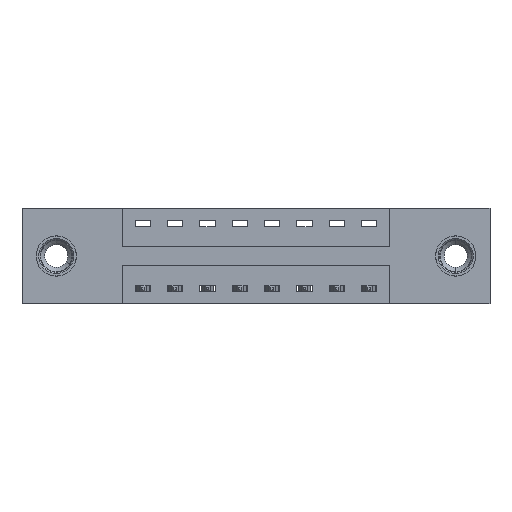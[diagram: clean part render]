
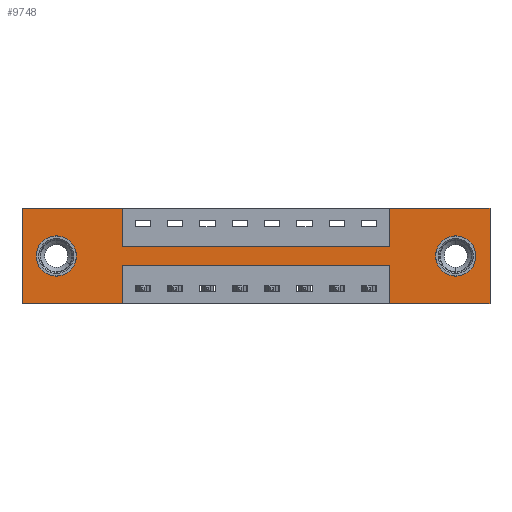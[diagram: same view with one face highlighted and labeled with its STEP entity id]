
A CAD part, front view. The second image highlights one B-rep face of the part: STEP entity #9748.
In plain terms, the highlighted planar face has unit normal (0, -1, 0).
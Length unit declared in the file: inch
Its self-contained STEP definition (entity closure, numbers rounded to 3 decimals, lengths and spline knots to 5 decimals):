
#38 = VERTEX_POINT ( 'NONE', #6421 ) ;
#64 = EDGE_LOOP ( 'NONE', ( #5988, #2363 ) ) ;
#204 = LINE ( 'NONE', #2705, #6734 ) ;
#238 = CARTESIAN_POINT ( 'NONE',  ( 0.3875, 0., -0.22 ) ) ;
#271 = LINE ( 'NONE', #597, #4645 ) ;
#382 = ORIENTED_EDGE ( 'NONE', *, *, #5666, .F. ) ;
#433 = EDGE_CURVE ( 'NONE', #2110, #8486, #7296, .T. ) ;
#437 = CARTESIAN_POINT ( 'NONE',  ( 0., 0., 0. ) ) ;
#597 = CARTESIAN_POINT ( 'NONE',  ( 0.3875, 0., -0.37 ) ) ;
#605 = CARTESIAN_POINT ( 'NONE',  ( 1.6775, 0., -0.185 ) ) ;
#645 = LINE ( 'NONE', #3397, #930 ) ;
#767 = EDGE_CURVE ( 'NONE', #38, #3267, #10589, .T. ) ;
#905 = VERTEX_POINT ( 'NONE', #4752 ) ;
#921 = ORIENTED_EDGE ( 'NONE', *, *, #1501, .F. ) ;
#930 = VECTOR ( 'NONE', #9151, 39.37008 ) ;
#946 = ORIENTED_EDGE ( 'NONE', *, *, #3650, .F. ) ;
#1101 = VECTOR ( 'NONE', #7994, 39.37008 ) ;
#1183 = VERTEX_POINT ( 'NONE', #7125 ) ;
#1222 = AXIS2_PLACEMENT_3D ( 'NONE', #1968, #10195, #5413 ) ;
#1232 = VECTOR ( 'NONE', #1485, 39.37008 ) ;
#1287 = AXIS2_PLACEMENT_3D ( 'NONE', #2606, #8405, #3456 ) ;
#1337 = ORIENTED_EDGE ( 'NONE', *, *, #9302, .F. ) ;
#1341 = FACE_BOUND ( 'NONE', #9958, .T. ) ;
#1353 = CARTESIAN_POINT ( 'NONE',  ( 1.81, 0., 0. ) ) ;
#1474 = ORIENTED_EDGE ( 'NONE', *, *, #5141, .F. ) ;
#1485 = DIRECTION ( 'NONE',  ( 1., 0., 0. ) ) ;
#1493 = DIRECTION ( 'NONE',  ( 0., 0., -1. ) ) ;
#1501 = EDGE_CURVE ( 'NONE', #9305, #10160, #5220, .T. ) ;
#1562 = CARTESIAN_POINT ( 'NONE',  ( 0.3875, 0., -0.22 ) ) ;
#1576 = VERTEX_POINT ( 'NONE', #10433 ) ;
#1651 = VECTOR ( 'NONE', #6190, 39.37008 ) ;
#1661 = AXIS2_PLACEMENT_3D ( 'NONE', #4784, #10378, #5609 ) ;
#1804 = DIRECTION ( 'NONE',  ( 0., 0., 1. ) ) ;
#1968 = CARTESIAN_POINT ( 'NONE',  ( 0., 0., -0.37 ) ) ;
#2008 = ORIENTED_EDGE ( 'NONE', *, *, #767, .F. ) ;
#2110 = VERTEX_POINT ( 'NONE', #6251 ) ;
#2145 = CARTESIAN_POINT ( 'NONE',  ( 1.4225, 0., -0.37 ) ) ;
#2183 = ORIENTED_EDGE ( 'NONE', *, *, #8426, .F. ) ;
#2271 = DIRECTION ( 'NONE',  ( 1., 0., 0. ) ) ;
#2363 = ORIENTED_EDGE ( 'NONE', *, *, #6330, .T. ) ;
#2386 = CARTESIAN_POINT ( 'NONE',  ( 1.4225, 0., -0.22 ) ) ;
#2452 = VERTEX_POINT ( 'NONE', #8284 ) ;
#2469 = DIRECTION ( 'NONE',  ( 0., 1., 0. ) ) ;
#2606 = CARTESIAN_POINT ( 'NONE',  ( 0.1325, 0., -0.185 ) ) ;
#2697 = VERTEX_POINT ( 'NONE', #9486 ) ;
#2705 = CARTESIAN_POINT ( 'NONE',  ( 0., 0., 0. ) ) ;
#2707 = CARTESIAN_POINT ( 'NONE',  ( 0.3875, 0., 0. ) ) ;
#2817 = CIRCLE ( 'NONE', #1661, 0.078 ) ;
#2905 = ORIENTED_EDGE ( 'NONE', *, *, #5493, .F. ) ;
#3236 = EDGE_CURVE ( 'NONE', #1576, #4786, #9096, .T. ) ;
#3246 = AXIS2_PLACEMENT_3D ( 'NONE', #7494, #2469, #8277 ) ;
#3267 = VERTEX_POINT ( 'NONE', #7894 ) ;
#3397 = CARTESIAN_POINT ( 'NONE',  ( 1.4225, 0., 0. ) ) ;
#3455 = VECTOR ( 'NONE', #5183, 39.37008 ) ;
#3456 = DIRECTION ( 'NONE',  ( 0., 0., 1. ) ) ;
#3497 = EDGE_CURVE ( 'NONE', #2697, #905, #6804, .T. ) ;
#3650 = EDGE_CURVE ( 'NONE', #10160, #2110, #5708, .T. ) ;
#3912 = CARTESIAN_POINT ( 'NONE',  ( 0., 0., -0.37 ) ) ;
#4524 = VECTOR ( 'NONE', #4642, 39.37008 ) ;
#4527 = CARTESIAN_POINT ( 'NONE',  ( 0., 0., -0.37 ) ) ;
#4559 = VECTOR ( 'NONE', #6404, 39.37008 ) ;
#4587 = PLANE ( 'NONE',  #1222 ) ;
#4642 = DIRECTION ( 'NONE',  ( -1., 0., 0. ) ) ;
#4645 = VECTOR ( 'NONE', #10512, 39.37008 ) ;
#4752 = CARTESIAN_POINT ( 'NONE',  ( 1.6775, 0., -0.263 ) ) ;
#4784 = CARTESIAN_POINT ( 'NONE',  ( 0.1325, 0., -0.185 ) ) ;
#4786 = VERTEX_POINT ( 'NONE', #4527 ) ;
#5141 = EDGE_CURVE ( 'NONE', #10484, #1576, #271, .T. ) ;
#5183 = DIRECTION ( 'NONE',  ( 0., 0., -1. ) ) ;
#5215 = EDGE_CURVE ( 'NONE', #1183, #6131, #8218, .T. ) ;
#5220 = LINE ( 'NONE', #6111, #9248 ) ;
#5273 = CARTESIAN_POINT ( 'NONE',  ( 0.3875, 0., -0.15 ) ) ;
#5409 = EDGE_CURVE ( 'NONE', #6879, #10484, #6156, .T. ) ;
#5413 = DIRECTION ( 'NONE',  ( 0., 0., -1. ) ) ;
#5493 = EDGE_CURVE ( 'NONE', #2452, #6879, #7342, .T. ) ;
#5609 = DIRECTION ( 'NONE',  ( 0., 0., 1. ) ) ;
#5666 = EDGE_CURVE ( 'NONE', #7062, #38, #10026, .T. ) ;
#5708 = LINE ( 'NONE', #9967, #3455 ) ;
#5742 = ORIENTED_EDGE ( 'NONE', *, *, #433, .F. ) ;
#5788 = CIRCLE ( 'NONE', #3246, 0.078 ) ;
#5881 = FACE_OUTER_BOUND ( 'NONE', #9182, .T. ) ;
#5988 = ORIENTED_EDGE ( 'NONE', *, *, #3497, .T. ) ;
#6099 = CARTESIAN_POINT ( 'NONE',  ( 1.4225, 0., -0.15 ) ) ;
#6111 = CARTESIAN_POINT ( 'NONE',  ( 0., 0., 0. ) ) ;
#6131 = VERTEX_POINT ( 'NONE', #8785 ) ;
#6156 = LINE ( 'NONE', #238, #1651 ) ;
#6190 = DIRECTION ( 'NONE',  ( -1., 0., 0. ) ) ;
#6251 = CARTESIAN_POINT ( 'NONE',  ( 0.3875, 0., -0.15 ) ) ;
#6330 = EDGE_CURVE ( 'NONE', #905, #2697, #5788, .T. ) ;
#6404 = DIRECTION ( 'NONE',  ( -1., 0., 0. ) ) ;
#6421 = CARTESIAN_POINT ( 'NONE',  ( 1.81, 0., 0. ) ) ;
#6560 = DIRECTION ( 'NONE',  ( 0., 1., 0. ) ) ;
#6716 = LINE ( 'NONE', #3912, #4559 ) ;
#6734 = VECTOR ( 'NONE', #1804, 39.37008 ) ;
#6804 = CIRCLE ( 'NONE', #8490, 0.078 ) ;
#6826 = ORIENTED_EDGE ( 'NONE', *, *, #9295, .T. ) ;
#6879 = VERTEX_POINT ( 'NONE', #2386 ) ;
#7062 = VERTEX_POINT ( 'NONE', #7681 ) ;
#7125 = CARTESIAN_POINT ( 'NONE',  ( 0.1325, 0., -0.263 ) ) ;
#7296 = LINE ( 'NONE', #5273, #7792 ) ;
#7342 = LINE ( 'NONE', #2145, #1101 ) ;
#7401 = CARTESIAN_POINT ( 'NONE',  ( 0., 0., 0. ) ) ;
#7494 = CARTESIAN_POINT ( 'NONE',  ( 1.6775, 0., -0.185 ) ) ;
#7681 = CARTESIAN_POINT ( 'NONE',  ( 1.4225, 0., 0. ) ) ;
#7792 = VECTOR ( 'NONE', #2271, 39.37008 ) ;
#7894 = CARTESIAN_POINT ( 'NONE',  ( 1.81, 0., -0.37 ) ) ;
#7994 = DIRECTION ( 'NONE',  ( 0., 0., 1. ) ) ;
#8218 = CIRCLE ( 'NONE', #1287, 0.078 ) ;
#8277 = DIRECTION ( 'NONE',  ( 0., 0., -1. ) ) ;
#8284 = CARTESIAN_POINT ( 'NONE',  ( 1.4225, 0., -0.37 ) ) ;
#8405 = DIRECTION ( 'NONE',  ( 0., 1., 0. ) ) ;
#8421 = DIRECTION ( 'NONE',  ( 1., 0., 0. ) ) ;
#8426 = EDGE_CURVE ( 'NONE', #4786, #9305, #204, .T. ) ;
#8486 = VERTEX_POINT ( 'NONE', #6099 ) ;
#8490 = AXIS2_PLACEMENT_3D ( 'NONE', #605, #6560, #1493 ) ;
#8524 = DIRECTION ( 'NONE',  ( 0., 0., -1. ) ) ;
#8532 = VECTOR ( 'NONE', #8524, 39.37008 ) ;
#8696 = CARTESIAN_POINT ( 'NONE',  ( 0., 0., -0.37 ) ) ;
#8785 = CARTESIAN_POINT ( 'NONE',  ( 0.1325, 0., -0.107 ) ) ;
#8843 = ORIENTED_EDGE ( 'NONE', *, *, #10047, .F. ) ;
#9096 = LINE ( 'NONE', #8696, #4524 ) ;
#9151 = DIRECTION ( 'NONE',  ( 0., 0., 1. ) ) ;
#9182 = EDGE_LOOP ( 'NONE', ( #1474, #10635, #2905, #1337, #2008, #382, #8843, #5742, #946, #921, #2183, #9616 ) ) ;
#9248 = VECTOR ( 'NONE', #8421, 39.37008 ) ;
#9295 = EDGE_CURVE ( 'NONE', #6131, #1183, #2817, .T. ) ;
#9302 = EDGE_CURVE ( 'NONE', #3267, #2452, #6716, .T. ) ;
#9305 = VERTEX_POINT ( 'NONE', #437 ) ;
#9486 = CARTESIAN_POINT ( 'NONE',  ( 1.6775, 0., -0.107 ) ) ;
#9616 = ORIENTED_EDGE ( 'NONE', *, *, #3236, .F. ) ;
#9748 = ADVANCED_FACE ( 'NONE', ( #10123, #1341, #5881 ), #4587, .T. ) ;
#9888 = ORIENTED_EDGE ( 'NONE', *, *, #5215, .T. ) ;
#9958 = EDGE_LOOP ( 'NONE', ( #6826, #9888 ) ) ;
#9967 = CARTESIAN_POINT ( 'NONE',  ( 0.3875, 0., 0. ) ) ;
#10026 = LINE ( 'NONE', #7401, #1232 ) ;
#10047 = EDGE_CURVE ( 'NONE', #8486, #7062, #645, .T. ) ;
#10123 = FACE_BOUND ( 'NONE', #64, .T. ) ;
#10160 = VERTEX_POINT ( 'NONE', #2707 ) ;
#10195 = DIRECTION ( 'NONE',  ( 0., -1., 0. ) ) ;
#10378 = DIRECTION ( 'NONE',  ( 0., 1., 0. ) ) ;
#10433 = CARTESIAN_POINT ( 'NONE',  ( 0.3875, 0., -0.37 ) ) ;
#10484 = VERTEX_POINT ( 'NONE', #1562 ) ;
#10512 = DIRECTION ( 'NONE',  ( 0., 0., -1. ) ) ;
#10589 = LINE ( 'NONE', #1353, #8532 ) ;
#10635 = ORIENTED_EDGE ( 'NONE', *, *, #5409, .F. ) ;
